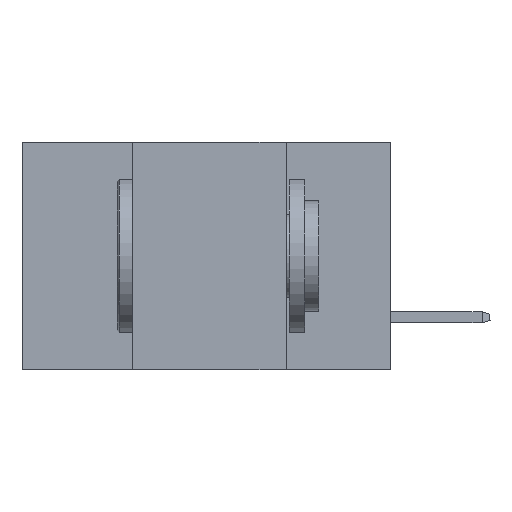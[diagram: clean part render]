
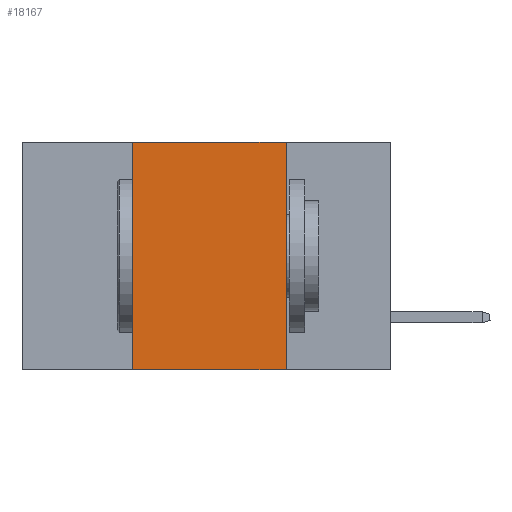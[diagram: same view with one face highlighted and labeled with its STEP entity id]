
A CAD part, left-side view. The second image highlights one B-rep face of the part: STEP entity #18167.
In plain terms, the highlighted planar face has unit normal (-1, 0, 0).
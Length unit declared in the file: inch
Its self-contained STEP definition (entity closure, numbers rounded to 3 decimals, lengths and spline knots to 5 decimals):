
#369 = VECTOR ( 'NONE', #8351, 39.37008 ) ;
#829 = CARTESIAN_POINT ( 'NONE',  ( 0., 0.42, 0. ) ) ;
#892 = CARTESIAN_POINT ( 'NONE',  ( 0., 0.42, -0.37 ) ) ;
#984 = PLANE ( 'NONE',  #3231 ) ;
#1116 = LINE ( 'NONE', #17434, #10606 ) ;
#1476 = DIRECTION ( 'NONE',  ( 0., -1., 0. ) ) ;
#2121 = DIRECTION ( 'NONE',  ( 0., 0., -1. ) ) ;
#2502 = ORIENTED_EDGE ( 'NONE', *, *, #8548, .F. ) ;
#3231 = AXIS2_PLACEMENT_3D ( 'NONE', #8553, #5763, #2121 ) ;
#3273 = FACE_OUTER_BOUND ( 'NONE', #10195, .T. ) ;
#4384 = CARTESIAN_POINT ( 'NONE',  ( 0., 0.17, 0. ) ) ;
#4397 = EDGE_CURVE ( 'NONE', #18057, #9128, #15967, .T. ) ;
#4791 = DIRECTION ( 'NONE',  ( 0., 0., -1. ) ) ;
#5763 = DIRECTION ( 'NONE',  ( 1., 0., 0. ) ) ;
#6337 = CARTESIAN_POINT ( 'NONE',  ( 0., 0.6, -0.37 ) ) ;
#6499 = EDGE_CURVE ( 'NONE', #17856, #9128, #1116, .T. ) ;
#7469 = ORIENTED_EDGE ( 'NONE', *, *, #6499, .F. ) ;
#7603 = VECTOR ( 'NONE', #16139, 39.37008 ) ;
#8114 = VECTOR ( 'NONE', #1476, 39.37008 ) ;
#8351 = DIRECTION ( 'NONE',  ( 0., 0., 1. ) ) ;
#8548 = EDGE_CURVE ( 'NONE', #18057, #8725, #12521, .T. ) ;
#8553 = CARTESIAN_POINT ( 'NONE',  ( 0., 0.6, 0. ) ) ;
#8725 = VERTEX_POINT ( 'NONE', #829 ) ;
#9128 = VERTEX_POINT ( 'NONE', #14250 ) ;
#9830 = EDGE_CURVE ( 'NONE', #8725, #17856, #15377, .T. ) ;
#10195 = EDGE_LOOP ( 'NONE', ( #7469, #10735, #2502, #11162 ) ) ;
#10606 = VECTOR ( 'NONE', #4791, 39.37008 ) ;
#10735 = ORIENTED_EDGE ( 'NONE', *, *, #9830, .F. ) ;
#11162 = ORIENTED_EDGE ( 'NONE', *, *, #4397, .T. ) ;
#12521 = LINE ( 'NONE', #13944, #369 ) ;
#13944 = CARTESIAN_POINT ( 'NONE',  ( 0., 0.42, 0. ) ) ;
#14164 = CARTESIAN_POINT ( 'NONE',  ( 0., 0.6, 0. ) ) ;
#14250 = CARTESIAN_POINT ( 'NONE',  ( 0., 0.17, -0.37 ) ) ;
#15377 = LINE ( 'NONE', #14164, #8114 ) ;
#15967 = LINE ( 'NONE', #6337, #7603 ) ;
#16139 = DIRECTION ( 'NONE',  ( 0., -1., 0. ) ) ;
#17434 = CARTESIAN_POINT ( 'NONE',  ( 0., 0.17, 0. ) ) ;
#17856 = VERTEX_POINT ( 'NONE', #4384 ) ;
#18057 = VERTEX_POINT ( 'NONE', #892 ) ;
#18167 = ADVANCED_FACE ( 'NONE', ( #3273 ), #984, .F. ) ;
